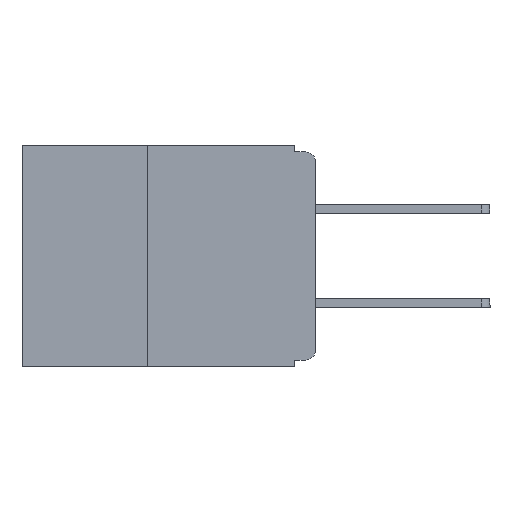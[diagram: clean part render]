
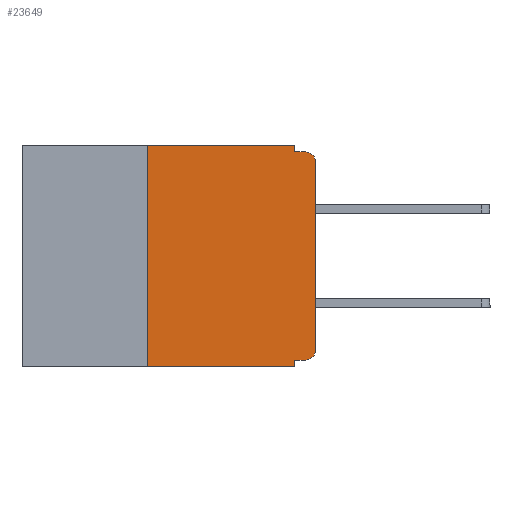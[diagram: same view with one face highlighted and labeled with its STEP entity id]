
A CAD part, left-side view. The second image highlights one B-rep face of the part: STEP entity #23649.
In plain terms, the highlighted planar face has unit normal (-1, 0, 0).
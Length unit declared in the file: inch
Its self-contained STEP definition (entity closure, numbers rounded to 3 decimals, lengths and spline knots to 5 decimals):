
#278 = VECTOR ( 'NONE', #18017, 39.37008 ) ;
#591 = VECTOR ( 'NONE', #23694, 39.37008 ) ;
#619 = VERTEX_POINT ( 'NONE', #12759 ) ;
#1147 = CARTESIAN_POINT ( 'NONE',  ( 0., 0.031, -0.32 ) ) ;
#2171 = AXIS2_PLACEMENT_3D ( 'NONE', #17497, #17401, #17397 ) ;
#2481 = VERTEX_POINT ( 'NONE', #5953 ) ;
#2590 = LINE ( 'NONE', #15767, #21506 ) ;
#2849 = DIRECTION ( 'NONE',  ( 0., 0., -1. ) ) ;
#2878 = DIRECTION ( 'NONE',  ( -1., 0., 0. ) ) ;
#2961 = CARTESIAN_POINT ( 'NONE',  ( 0., 0.015, -0.025 ) ) ;
#3111 = LINE ( 'NONE', #9469, #17645 ) ;
#3450 = VERTEX_POINT ( 'NONE', #1147 ) ;
#3652 = EDGE_CURVE ( 'NONE', #7771, #16598, #12764, .T. ) ;
#4265 = EDGE_CURVE ( 'NONE', #3450, #10225, #15101, .T. ) ;
#4301 = LINE ( 'NONE', #7161, #13222 ) ;
#4444 = EDGE_CURVE ( 'NONE', #16598, #13498, #5913, .T. ) ;
#4660 = PLANE ( 'NONE',  #18936 ) ;
#4667 = FACE_OUTER_BOUND ( 'NONE', #19745, .T. ) ;
#4728 = AXIS2_PLACEMENT_3D ( 'NONE', #2961, #2878, #2849 ) ;
#5017 = VECTOR ( 'NONE', #14265, 39.37008 ) ;
#5096 = EDGE_CURVE ( 'NONE', #2481, #619, #20648, .T. ) ;
#5522 = EDGE_CURVE ( 'NONE', #19978, #10225, #15635, .T. ) ;
#5643 = LINE ( 'NONE', #14182, #5017 ) ;
#5913 = LINE ( 'NONE', #18275, #278 ) ;
#5953 = CARTESIAN_POINT ( 'NONE',  ( 0., 0.25, 0. ) ) ;
#6154 = VECTOR ( 'NONE', #19468, 39.37008 ) ;
#6200 = EDGE_CURVE ( 'NONE', #13498, #8667, #20290, .T. ) ;
#6413 = CARTESIAN_POINT ( 'NONE',  ( 0., 0.031, -0.01 ) ) ;
#7161 = CARTESIAN_POINT ( 'NONE',  ( 0., 0., -0.32 ) ) ;
#7771 = VERTEX_POINT ( 'NONE', #14770 ) ;
#8112 = EDGE_CURVE ( 'NONE', #19978, #2481, #2590, .T. ) ;
#8536 = DIRECTION ( 'NONE',  ( 1., 0., 0. ) ) ;
#8667 = VERTEX_POINT ( 'NONE', #23054 ) ;
#8775 = CARTESIAN_POINT ( 'NONE',  ( 0., 0., -0.025 ) ) ;
#9387 = EDGE_CURVE ( 'NONE', #619, #13833, #3111, .T. ) ;
#9469 = CARTESIAN_POINT ( 'NONE',  ( 0., 0.031, 0. ) ) ;
#10225 = VERTEX_POINT ( 'NONE', #13805 ) ;
#12094 = DIRECTION ( 'NONE',  ( 0., 0., 1. ) ) ;
#12759 = CARTESIAN_POINT ( 'NONE',  ( 0., 0.031, 0. ) ) ;
#12764 = CIRCLE ( 'NONE', #2171, 0.015 ) ;
#13222 = VECTOR ( 'NONE', #22213, 39.37008 ) ;
#13498 = VERTEX_POINT ( 'NONE', #8775 ) ;
#13805 = CARTESIAN_POINT ( 'NONE',  ( 0., 0.031, -0.33 ) ) ;
#13833 = VERTEX_POINT ( 'NONE', #6413 ) ;
#13991 = ORIENTED_EDGE ( 'NONE', *, *, #22603, .F. ) ;
#14182 = CARTESIAN_POINT ( 'NONE',  ( 0., 0., -0.01 ) ) ;
#14265 = DIRECTION ( 'NONE',  ( 0., -1., 0. ) ) ;
#14770 = CARTESIAN_POINT ( 'NONE',  ( 0., 0.015, -0.32 ) ) ;
#15075 = EDGE_CURVE ( 'NONE', #7771, #3450, #4301, .T. ) ;
#15101 = LINE ( 'NONE', #23446, #591 ) ;
#15635 = LINE ( 'NONE', #19595, #6154 ) ;
#15767 = CARTESIAN_POINT ( 'NONE',  ( 0., 0.25, -0.33 ) ) ;
#15846 = ORIENTED_EDGE ( 'NONE', *, *, #4444, .T. ) ;
#16598 = VERTEX_POINT ( 'NONE', #18905 ) ;
#16601 = ORIENTED_EDGE ( 'NONE', *, *, #9387, .F. ) ;
#17052 = DIRECTION ( 'NONE',  ( 0., 0., -1. ) ) ;
#17099 = ORIENTED_EDGE ( 'NONE', *, *, #5096, .F. ) ;
#17397 = DIRECTION ( 'NONE',  ( 0., 0., -1. ) ) ;
#17401 = DIRECTION ( 'NONE',  ( -1., 0., 0. ) ) ;
#17497 = CARTESIAN_POINT ( 'NONE',  ( 0., 0.015, -0.305 ) ) ;
#17645 = VECTOR ( 'NONE', #17052, 39.37008 ) ;
#18017 = DIRECTION ( 'NONE',  ( 0., 0., 1. ) ) ;
#18136 = ORIENTED_EDGE ( 'NONE', *, *, #6200, .T. ) ;
#18275 = CARTESIAN_POINT ( 'NONE',  ( 0., 0., 0. ) ) ;
#18561 = ORIENTED_EDGE ( 'NONE', *, *, #4265, .F. ) ;
#18615 = ORIENTED_EDGE ( 'NONE', *, *, #8112, .F. ) ;
#18905 = CARTESIAN_POINT ( 'NONE',  ( 0., 0., -0.305 ) ) ;
#18936 = AXIS2_PLACEMENT_3D ( 'NONE', #19815, #8536, #21680 ) ;
#19100 = DIRECTION ( 'NONE',  ( 0., -1., 0. ) ) ;
#19157 = CARTESIAN_POINT ( 'NONE',  ( 0., 0.437, 0. ) ) ;
#19468 = DIRECTION ( 'NONE',  ( 0., -1., 0. ) ) ;
#19485 = CARTESIAN_POINT ( 'NONE',  ( 0., 0.25, -0.33 ) ) ;
#19595 = CARTESIAN_POINT ( 'NONE',  ( 0., 0.437, -0.33 ) ) ;
#19745 = EDGE_LOOP ( 'NONE', ( #15846, #18136, #13991, #16601, #17099, #18615, #22288, #18561, #24299, #21994 ) ) ;
#19815 = CARTESIAN_POINT ( 'NONE',  ( 0., 0.437, 0. ) ) ;
#19978 = VERTEX_POINT ( 'NONE', #19485 ) ;
#20290 = CIRCLE ( 'NONE', #4728, 0.015 ) ;
#20648 = LINE ( 'NONE', #19157, #24307 ) ;
#21506 = VECTOR ( 'NONE', #12094, 39.37008 ) ;
#21680 = DIRECTION ( 'NONE',  ( 0., 0., -1. ) ) ;
#21994 = ORIENTED_EDGE ( 'NONE', *, *, #3652, .T. ) ;
#22213 = DIRECTION ( 'NONE',  ( 0., 1., 0. ) ) ;
#22288 = ORIENTED_EDGE ( 'NONE', *, *, #5522, .T. ) ;
#22603 = EDGE_CURVE ( 'NONE', #13833, #8667, #5643, .T. ) ;
#23054 = CARTESIAN_POINT ( 'NONE',  ( 0., 0.015, -0.01 ) ) ;
#23446 = CARTESIAN_POINT ( 'NONE',  ( 0., 0.031, -0.33 ) ) ;
#23649 = ADVANCED_FACE ( 'NONE', ( #4667 ), #4660, .F. ) ;
#23694 = DIRECTION ( 'NONE',  ( 0., 0., -1. ) ) ;
#24299 = ORIENTED_EDGE ( 'NONE', *, *, #15075, .F. ) ;
#24307 = VECTOR ( 'NONE', #19100, 39.37008 ) ;
